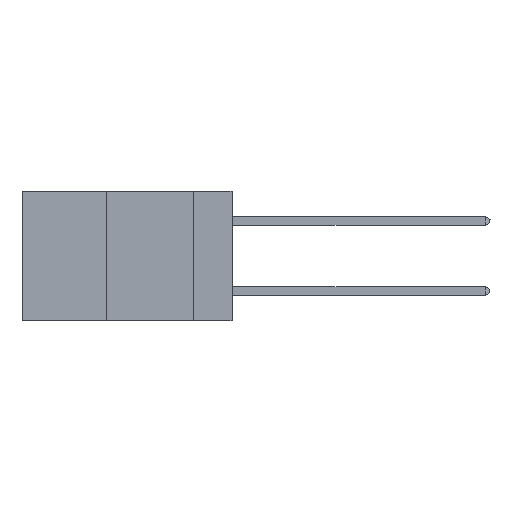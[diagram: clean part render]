
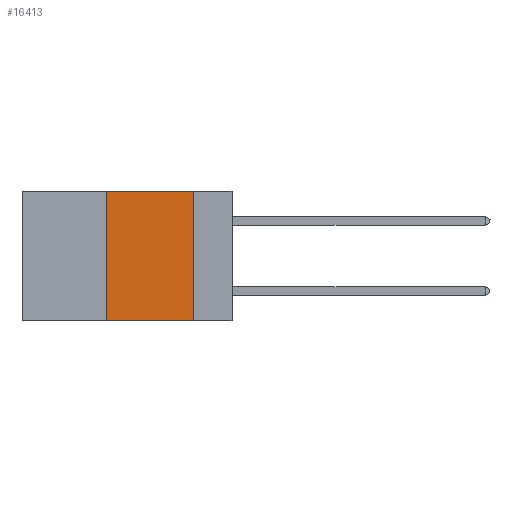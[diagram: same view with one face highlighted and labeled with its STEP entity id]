
A CAD part, left-side view. The second image highlights one B-rep face of the part: STEP entity #16413.
In plain terms, the highlighted planar face has unit normal (-1, 0, 0).
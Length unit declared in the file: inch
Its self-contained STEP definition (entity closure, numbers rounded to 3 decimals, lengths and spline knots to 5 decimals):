
#90 = EDGE_CURVE ( 'NONE', #1833, #857, #35001, .T. ) ;
#857 = VERTEX_POINT ( 'NONE', #9471 ) ;
#1833 = VERTEX_POINT ( 'NONE', #7287 ) ;
#1851 = DIRECTION ( 'NONE',  ( 0., 0., -1. ) ) ;
#3576 = EDGE_CURVE ( 'NONE', #1833, #33170, #4623, .T. ) ;
#4623 = LINE ( 'NONE', #7633, #19671 ) ;
#6853 = ORIENTED_EDGE ( 'NONE', *, *, #37824, .F. ) ;
#7000 = ORIENTED_EDGE ( 'NONE', *, *, #90, .T. ) ;
#7287 = CARTESIAN_POINT ( 'NONE',  ( 0., 0.36, -0.37 ) ) ;
#7633 = CARTESIAN_POINT ( 'NONE',  ( 0., 0.36, 0. ) ) ;
#7695 = CARTESIAN_POINT ( 'NONE',  ( 0., 0.6, 0. ) ) ;
#9471 = CARTESIAN_POINT ( 'NONE',  ( 0., 0.11, -0.37 ) ) ;
#10559 = CARTESIAN_POINT ( 'NONE',  ( 0., 0.6, -0.37 ) ) ;
#10919 = CARTESIAN_POINT ( 'NONE',  ( 0., 0.11, 0. ) ) ;
#11792 = ORIENTED_EDGE ( 'NONE', *, *, #14136, .F. ) ;
#13486 = DIRECTION ( 'NONE',  ( 0., 0., 1. ) ) ;
#13666 = FACE_OUTER_BOUND ( 'NONE', #14492, .T. ) ;
#13946 = LINE ( 'NONE', #10919, #33489 ) ;
#14136 = EDGE_CURVE ( 'NONE', #33170, #31247, #20609, .T. ) ;
#14492 = EDGE_LOOP ( 'NONE', ( #6853, #11792, #38331, #7000 ) ) ;
#16413 = ADVANCED_FACE ( 'NONE', ( #13666 ), #16476, .F. ) ;
#16476 = PLANE ( 'NONE',  #25832 ) ;
#16776 = DIRECTION ( 'NONE',  ( 0., -1., 0. ) ) ;
#19671 = VECTOR ( 'NONE', #13486, 39.37008 ) ;
#20609 = LINE ( 'NONE', #7695, #36339 ) ;
#22884 = DIRECTION ( 'NONE',  ( 0., -1., 0. ) ) ;
#24097 = DIRECTION ( 'NONE',  ( 1., 0., 0. ) ) ;
#25832 = AXIS2_PLACEMENT_3D ( 'NONE', #28791, #24097, #38086 ) ;
#28791 = CARTESIAN_POINT ( 'NONE',  ( 0., 0.6, 0. ) ) ;
#31247 = VERTEX_POINT ( 'NONE', #38391 ) ;
#33170 = VERTEX_POINT ( 'NONE', #34697 ) ;
#33489 = VECTOR ( 'NONE', #1851, 39.37008 ) ;
#34697 = CARTESIAN_POINT ( 'NONE',  ( 0., 0.36, 0. ) ) ;
#35001 = LINE ( 'NONE', #10559, #35337 ) ;
#35337 = VECTOR ( 'NONE', #22884, 39.37008 ) ;
#36339 = VECTOR ( 'NONE', #16776, 39.37008 ) ;
#37824 = EDGE_CURVE ( 'NONE', #31247, #857, #13946, .T. ) ;
#38086 = DIRECTION ( 'NONE',  ( 0., 0., -1. ) ) ;
#38331 = ORIENTED_EDGE ( 'NONE', *, *, #3576, .F. ) ;
#38391 = CARTESIAN_POINT ( 'NONE',  ( 0., 0.11, 0. ) ) ;
